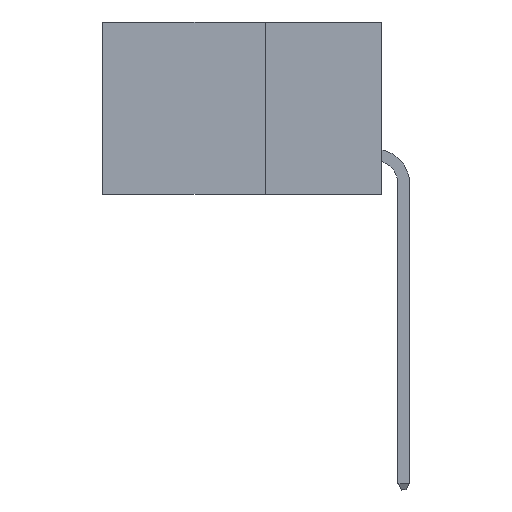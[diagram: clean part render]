
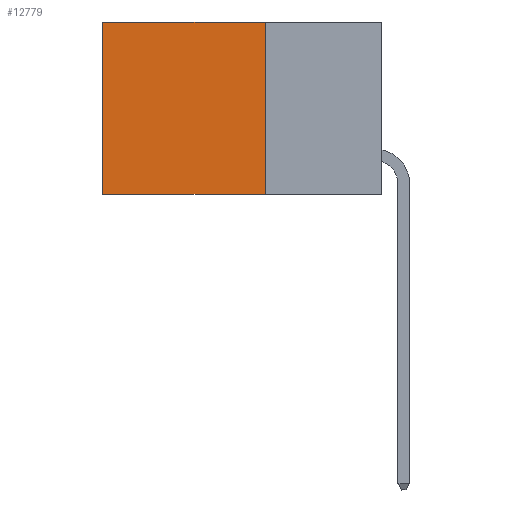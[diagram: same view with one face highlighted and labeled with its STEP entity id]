
A CAD part, left-side view. The second image highlights one B-rep face of the part: STEP entity #12779.
In plain terms, the highlighted planar face has unit normal (-1, 0, 0).
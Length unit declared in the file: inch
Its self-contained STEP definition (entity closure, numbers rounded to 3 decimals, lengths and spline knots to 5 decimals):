
#241 = AXIS2_PLACEMENT_3D ( 'NONE', #14537, #4464, #4922 ) ;
#369 = CARTESIAN_POINT ( 'NONE',  ( 0.2875, 0.6, 0. ) ) ;
#578 = VERTEX_POINT ( 'NONE', #7150 ) ;
#2114 = ORIENTED_EDGE ( 'NONE', *, *, #2772, .T. ) ;
#2590 = EDGE_CURVE ( 'NONE', #578, #8328, #14140, .T. ) ;
#2772 = EDGE_CURVE ( 'NONE', #13449, #8328, #19409, .T. ) ;
#4452 = CARTESIAN_POINT ( 'NONE',  ( 0.2875, 0.25, 0. ) ) ;
#4464 = DIRECTION ( 'NONE',  ( 1., 0., 0. ) ) ;
#4922 = DIRECTION ( 'NONE',  ( 0., 0., -1. ) ) ;
#4993 = PLANE ( 'NONE',  #241 ) ;
#5870 = ORIENTED_EDGE ( 'NONE', *, *, #20046, .T. ) ;
#7150 = CARTESIAN_POINT ( 'NONE',  ( 0.2875, 0.25, -0.37 ) ) ;
#8026 = VECTOR ( 'NONE', #9890, 39.37008 ) ;
#8328 = VERTEX_POINT ( 'NONE', #21533 ) ;
#8963 = LINE ( 'NONE', #13272, #11085 ) ;
#9570 = VERTEX_POINT ( 'NONE', #4452 ) ;
#9890 = DIRECTION ( 'NONE',  ( 0., 0., -1. ) ) ;
#10996 = EDGE_CURVE ( 'NONE', #9570, #578, #20141, .T. ) ;
#11085 = VECTOR ( 'NONE', #14968, 39.37008 ) ;
#11639 = DIRECTION ( 'NONE',  ( 0., 1., 0. ) ) ;
#12023 = VECTOR ( 'NONE', #11639, 39.37008 ) ;
#12779 = ADVANCED_FACE ( 'NONE', ( #12994 ), #4993, .F. ) ;
#12994 = FACE_OUTER_BOUND ( 'NONE', #20747, .T. ) ;
#13272 = CARTESIAN_POINT ( 'NONE',  ( 0.2875, 0.25, 0. ) ) ;
#13449 = VERTEX_POINT ( 'NONE', #19522 ) ;
#13690 = DIRECTION ( 'NONE',  ( 0., 0., -1. ) ) ;
#14140 = LINE ( 'NONE', #20109, #12023 ) ;
#14537 = CARTESIAN_POINT ( 'NONE',  ( 0.2875, 0.25, 0. ) ) ;
#14968 = DIRECTION ( 'NONE',  ( 0., 1., 0. ) ) ;
#16612 = ORIENTED_EDGE ( 'NONE', *, *, #2590, .F. ) ;
#16738 = VECTOR ( 'NONE', #13690, 39.37008 ) ;
#16788 = CARTESIAN_POINT ( 'NONE',  ( 0.2875, 0.25, 0. ) ) ;
#19409 = LINE ( 'NONE', #369, #16738 ) ;
#19522 = CARTESIAN_POINT ( 'NONE',  ( 0.2875, 0.6, 0. ) ) ;
#20046 = EDGE_CURVE ( 'NONE', #9570, #13449, #8963, .T. ) ;
#20109 = CARTESIAN_POINT ( 'NONE',  ( 0.2875, 0.25, -0.37 ) ) ;
#20141 = LINE ( 'NONE', #16788, #8026 ) ;
#20747 = EDGE_LOOP ( 'NONE', ( #2114, #16612, #21109, #5870 ) ) ;
#21109 = ORIENTED_EDGE ( 'NONE', *, *, #10996, .F. ) ;
#21533 = CARTESIAN_POINT ( 'NONE',  ( 0.2875, 0.6, -0.37 ) ) ;
